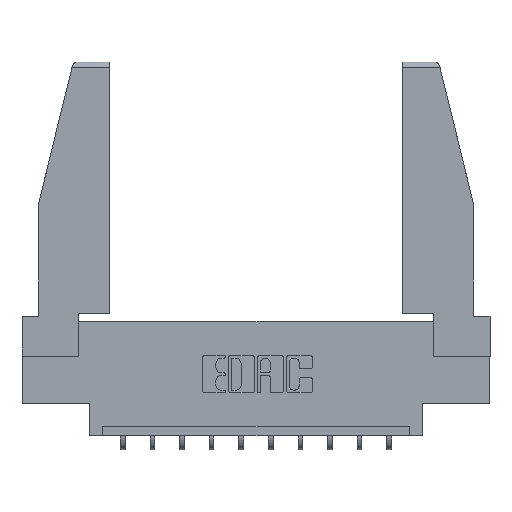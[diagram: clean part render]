
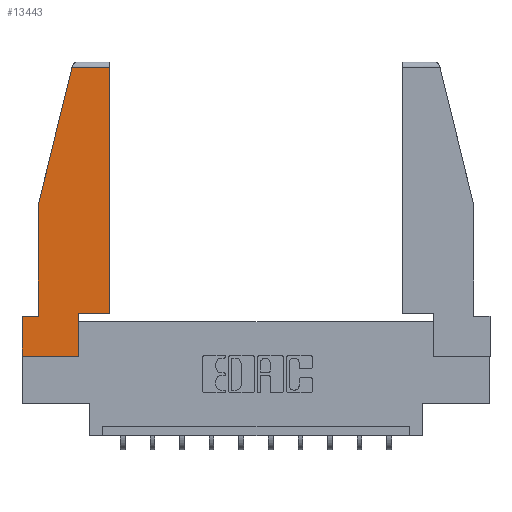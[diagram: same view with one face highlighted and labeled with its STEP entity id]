
A CAD part, top view. The second image highlights one B-rep face of the part: STEP entity #13443.
In plain terms, the highlighted planar face has unit normal (0, 0, 1).
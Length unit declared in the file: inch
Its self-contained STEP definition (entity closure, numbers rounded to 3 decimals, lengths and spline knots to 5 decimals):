
#76 = LINE ( 'NONE', #7154, #6964 ) ;
#114 = CARTESIAN_POINT ( 'NONE',  ( 0., 0.21, 0. ) ) ;
#128 = ORIENTED_EDGE ( 'NONE', *, *, #5689, .T. ) ;
#385 = DIRECTION ( 'NONE',  ( 1., 0., 0. ) ) ;
#502 = EDGE_CURVE ( 'NONE', #10733, #2952, #13446, .T. ) ;
#1029 = LINE ( 'NONE', #12886, #14264 ) ;
#1171 = VERTEX_POINT ( 'NONE', #13415 ) ;
#1457 = CARTESIAN_POINT ( 'NONE',  ( 0., 0.21, 0. ) ) ;
#2046 = CARTESIAN_POINT ( 'NONE',  ( 0.086, 0.8, 0. ) ) ;
#2388 = VECTOR ( 'NONE', #6415, 39.37008 ) ;
#2500 = ORIENTED_EDGE ( 'NONE', *, *, #5726, .T. ) ;
#2513 = CARTESIAN_POINT ( 'NONE',  ( 0., 0., 0. ) ) ;
#2573 = VERTEX_POINT ( 'NONE', #10905 ) ;
#2759 = LINE ( 'NONE', #10457, #12701 ) ;
#2952 = VERTEX_POINT ( 'NONE', #2513 ) ;
#3010 = DIRECTION ( 'NONE',  ( 0., 1., 0. ) ) ;
#3054 = DIRECTION ( 'NONE',  ( 1., 0., 0. ) ) ;
#3091 = ORIENTED_EDGE ( 'NONE', *, *, #4167, .T. ) ;
#3386 = DIRECTION ( 'NONE',  ( 0., 1., 0. ) ) ;
#3670 = FACE_OUTER_BOUND ( 'NONE', #11786, .T. ) ;
#3872 = EDGE_CURVE ( 'NONE', #2573, #10123, #12487, .T. ) ;
#4167 = EDGE_CURVE ( 'NONE', #6382, #1171, #13345, .T. ) ;
#4660 = CARTESIAN_POINT ( 'NONE',  ( 0., 1.52, 0. ) ) ;
#4693 = VERTEX_POINT ( 'NONE', #8492 ) ;
#4719 = CARTESIAN_POINT ( 'NONE',  ( 0.297, 0., 0. ) ) ;
#5438 = VECTOR ( 'NONE', #3386, 39.37008 ) ;
#5486 = VERTEX_POINT ( 'NONE', #12315 ) ;
#5607 = DIRECTION ( 'NONE',  ( -1., 0., 0. ) ) ;
#5689 = EDGE_CURVE ( 'NONE', #8862, #2573, #7828, .T. ) ;
#5726 = EDGE_CURVE ( 'NONE', #5486, #10733, #76, .T. ) ;
#5912 = PLANE ( 'NONE',  #14238 ) ;
#6382 = VERTEX_POINT ( 'NONE', #4719 ) ;
#6415 = DIRECTION ( 'NONE',  ( 0., -1., 0. ) ) ;
#6429 = ORIENTED_EDGE ( 'NONE', *, *, #3872, .T. ) ;
#6671 = LINE ( 'NONE', #11878, #2388 ) ;
#6964 = VECTOR ( 'NONE', #9920, 39.37008 ) ;
#7154 = CARTESIAN_POINT ( 'NONE',  ( 0., 0.21, 0. ) ) ;
#7775 = DIRECTION ( 'NONE',  ( 0., -1., 0. ) ) ;
#7828 = LINE ( 'NONE', #4660, #12621 ) ;
#8331 = LINE ( 'NONE', #8853, #5438 ) ;
#8492 = CARTESIAN_POINT ( 'NONE',  ( 0.461, 0.223, 0. ) ) ;
#8584 = CARTESIAN_POINT ( 'NONE',  ( 0.271, 1.55, 0. ) ) ;
#8853 = CARTESIAN_POINT ( 'NONE',  ( 0.461, 0.223, 0. ) ) ;
#8862 = VERTEX_POINT ( 'NONE', #9785 ) ;
#8897 = EDGE_CURVE ( 'NONE', #4693, #8862, #8331, .T. ) ;
#9049 = CARTESIAN_POINT ( 'NONE',  ( 0., 0., 0. ) ) ;
#9069 = ORIENTED_EDGE ( 'NONE', *, *, #8897, .T. ) ;
#9321 = ORIENTED_EDGE ( 'NONE', *, *, #502, .T. ) ;
#9785 = CARTESIAN_POINT ( 'NONE',  ( 0.461, 1.52, 0. ) ) ;
#9920 = DIRECTION ( 'NONE',  ( -1., 0., 0. ) ) ;
#10095 = DIRECTION ( 'NONE',  ( 1., 0., 0. ) ) ;
#10123 = VERTEX_POINT ( 'NONE', #2046 ) ;
#10457 = CARTESIAN_POINT ( 'NONE',  ( 0., 0., 0. ) ) ;
#10681 = CARTESIAN_POINT ( 'NONE',  ( 0.297, 0., 0. ) ) ;
#10733 = VERTEX_POINT ( 'NONE', #1457 ) ;
#10905 = CARTESIAN_POINT ( 'NONE',  ( 0.2636, 1.52, 0. ) ) ;
#10944 = VECTOR ( 'NONE', #12993, 39.37008 ) ;
#11642 = VECTOR ( 'NONE', #3010, 39.37008 ) ;
#11679 = ORIENTED_EDGE ( 'NONE', *, *, #11858, .T. ) ;
#11745 = EDGE_CURVE ( 'NONE', #2952, #6382, #2759, .T. ) ;
#11786 = EDGE_LOOP ( 'NONE', ( #9069, #128, #6429, #13942, #2500, #9321, #13803, #3091, #11679 ) ) ;
#11858 = EDGE_CURVE ( 'NONE', #1171, #4693, #1029, .T. ) ;
#11878 = CARTESIAN_POINT ( 'NONE',  ( 0.086, 0.8, 0. ) ) ;
#12224 = VECTOR ( 'NONE', #7775, 39.37008 ) ;
#12315 = CARTESIAN_POINT ( 'NONE',  ( 0.086, 0.21, 0. ) ) ;
#12326 = EDGE_CURVE ( 'NONE', #10123, #5486, #6671, .T. ) ;
#12487 = LINE ( 'NONE', #8584, #10944 ) ;
#12621 = VECTOR ( 'NONE', #5607, 39.37008 ) ;
#12701 = VECTOR ( 'NONE', #385, 39.37008 ) ;
#12886 = CARTESIAN_POINT ( 'NONE',  ( 0.297, 0.223, 0. ) ) ;
#12993 = DIRECTION ( 'NONE',  ( -0.239, -0.971, 0. ) ) ;
#13345 = LINE ( 'NONE', #10681, #11642 ) ;
#13415 = CARTESIAN_POINT ( 'NONE',  ( 0.297, 0.223, 0. ) ) ;
#13443 = ADVANCED_FACE ( 'NONE', ( #3670 ), #5912, .T. ) ;
#13446 = LINE ( 'NONE', #114, #12224 ) ;
#13575 = DIRECTION ( 'NONE',  ( 0., 0., 1. ) ) ;
#13803 = ORIENTED_EDGE ( 'NONE', *, *, #11745, .T. ) ;
#13942 = ORIENTED_EDGE ( 'NONE', *, *, #12326, .T. ) ;
#14238 = AXIS2_PLACEMENT_3D ( 'NONE', #9049, #13575, #10095 ) ;
#14264 = VECTOR ( 'NONE', #3054, 39.37008 ) ;
